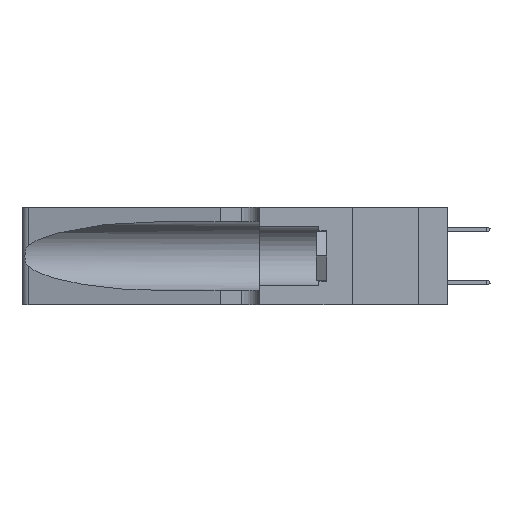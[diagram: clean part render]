
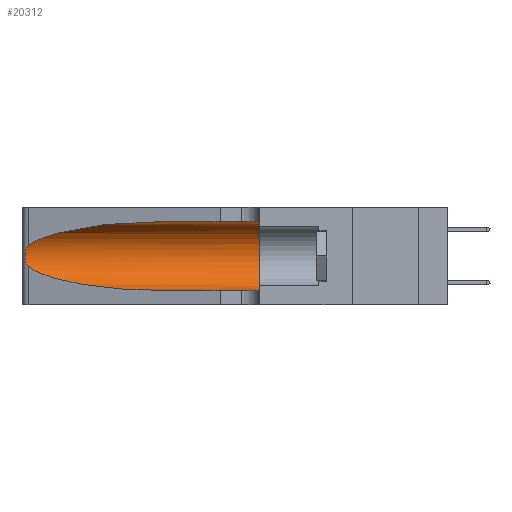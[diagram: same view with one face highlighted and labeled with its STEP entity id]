
A CAD part, left-side view. The second image highlights one B-rep face of the part: STEP entity #20312.
In plain terms, the highlighted cylindrical face has radius 3.308 mm (diameter 6.617 mm), a partial arc.
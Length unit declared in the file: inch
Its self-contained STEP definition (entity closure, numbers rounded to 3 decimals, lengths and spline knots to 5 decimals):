
#428 = VERTEX_POINT ( 'NONE', #33057 ) ;
#535 = ORIENTED_EDGE ( 'NONE', *, *, #45934, .F. ) ;
#1060 = CARTESIAN_POINT ( 'NONE',  ( 0.25639, 1.23186, 0.15144 ) ) ;
#3641 = CARTESIAN_POINT ( 'NONE',  ( 0.1305, 0.72297, 0.31525 ) ) ;
#3843 = LINE ( 'NONE', #36779, #40829 ) ;
#3960 = CARTESIAN_POINT ( 'NONE',  ( 0.1305, 0.35, 0.05475 ) ) ;
#4656 = CARTESIAN_POINT ( 'NONE',  ( 0.25639, 1.23184, 0.21858 ) ) ;
#4791 = VECTOR ( 'NONE', #8907, 39.37008 ) ;
#5279 = CARTESIAN_POINT ( 'NONE',  ( 0.25555, 1.22994, 0.2215 ) ) ;
#5611 = CARTESIAN_POINT ( 'NONE',  ( 0.18966, 0.96281, 0.31525 ) ) ;
#6118 = ORIENTED_EDGE ( 'NONE', *, *, #34752, .T. ) ;
#6640 = CARTESIAN_POINT ( 'NONE',  ( 0.1305, 0.35, 0.185 ) ) ;
#7784 = DIRECTION ( 'NONE',  ( 0., -1., 0. ) ) ;
#7878 = CARTESIAN_POINT ( 'NONE',  ( 0.25487, 1.22718, 0.14631 ) ) ;
#7932 = DIRECTION ( 'NONE',  ( 0., 0., -1. ) ) ;
#8340 = CARTESIAN_POINT ( 'NONE',  ( 0.1305, 0.72297, 0.05475 ) ) ;
#8907 = DIRECTION ( 'NONE',  ( 0., -1., 0. ) ) ;
#9810 = ORIENTED_EDGE ( 'NONE', *, *, #25348, .T. ) ;
#10190 = EDGE_LOOP ( 'NONE', ( #35758, #9810, #6118, #24271, #42509, #535 ) ) ;
#10231 = FACE_OUTER_BOUND ( 'NONE', #10190, .T. ) ;
#10929 = CARTESIAN_POINT ( 'NONE',  ( 0.1305, 0.72297, 0.05475 ) ) ;
#12458 = CARTESIAN_POINT ( 'NONE',  ( 0.25787, 1.23484, 0.2124 ) ) ;
#13278 = VERTEX_POINT ( 'NONE', #3641 ) ;
#15458 = CARTESIAN_POINT ( 'NONE',  ( 0.26075, 1.23896, 0.19203 ) ) ;
#15604 = CARTESIAN_POINT ( 'NONE',  ( 0.26075, 1.23896, 0.178 ) ) ;
#16070 = CARTESIAN_POINT ( 'NONE',  ( 0.25856, 1.23593, 0.16098 ) ) ;
#17024 = AXIS2_PLACEMENT_3D ( 'NONE', #6640, #39417, #32506 ) ;
#18526 = CARTESIAN_POINT ( 'NONE',  ( 0.2373, 1.15595, 0.08982 ) ) ;
#19727 = VERTEX_POINT ( 'NONE', #3960 ) ;
#20312 = ADVANCED_FACE ( 'NONE', ( #10231 ), #21423, .F. ) ;
#20934 = EDGE_CURVE ( 'NONE', #27615, #19727, #43351, .T. ) ;
#21423 = CYLINDRICAL_SURFACE ( 'NONE', #39854, 0.13025 ) ;
#22131 = CARTESIAN_POINT ( 'NONE',  ( 0.1305, 0.35, 0.31525 ) ) ;
#22502 = CARTESIAN_POINT ( 'NONE',  ( 0.25487, 1.22718, 0.14631 ) ) ;
#23610 = EDGE_CURVE ( 'NONE', #29507, #19727, #3843, .T. ) ;
#24271 = ORIENTED_EDGE ( 'NONE', *, *, #23610, .T. ) ;
#25348 = EDGE_CURVE ( 'NONE', #428, #28505, #37617, .T. ) ;
#26445 = CARTESIAN_POINT ( 'NONE',  ( 0.25487, 1.22718, 0.22369 ) ) ;
#26723 =( BOUNDED_CURVE ( )  B_SPLINE_CURVE ( 3, ( #7878, #18526, #44082, #8340 ),
 .UNSPECIFIED., .F., .F. ) 
 B_SPLINE_CURVE_WITH_KNOTS ( ( 4, 4 ),
 ( 3.44316, 4.71239 ),
 .UNSPECIFIED. ) 
 CURVE ( )  GEOMETRIC_REPRESENTATION_ITEM ( )  RATIONAL_B_SPLINE_CURVE ( ( 1., 0.87, 0.87, 1. ) ) 
 REPRESENTATION_ITEM ( '' )  );
#26768 = CARTESIAN_POINT ( 'NONE',  ( 0.26018, 1.23835, 0.19895 ) ) ;
#27615 = VERTEX_POINT ( 'NONE', #22131 ) ;
#28505 = VERTEX_POINT ( 'NONE', #44675 ) ;
#29507 = VERTEX_POINT ( 'NONE', #10929 ) ;
#30391 = CARTESIAN_POINT ( 'NONE',  ( 0.1305, 1.61858, 0.31525 ) ) ;
#32270 = LINE ( 'NONE', #30391, #4791 ) ;
#32506 = DIRECTION ( 'NONE',  ( 0., 0., 1. ) ) ;
#33057 = CARTESIAN_POINT ( 'NONE',  ( 0.25487, 1.22718, 0.22369 ) ) ;
#33923 = CARTESIAN_POINT ( 'NONE',  ( 0.26017, 1.23833, 0.17102 ) ) ;
#34752 = EDGE_CURVE ( 'NONE', #28505, #29507, #26723, .T. ) ;
#35692 = CARTESIAN_POINT ( 'NONE',  ( 0.1305, 1.61858, 0.185 ) ) ;
#35758 = ORIENTED_EDGE ( 'NONE', *, *, #40510, .T. ) ;
#36779 = CARTESIAN_POINT ( 'NONE',  ( 0.1305, 1.61858, 0.05475 ) ) ;
#36920 = CARTESIAN_POINT ( 'NONE',  ( 0.25854, 1.2359, 0.20912 ) ) ;
#37617 = B_SPLINE_CURVE_WITH_KNOTS ( 'NONE', 3,
 ( #26445, #5279, #4656, #12458, #36920, #26768, #15458, #15604, #33923, #16070, #43980, #1060, #40695, #22502 ),
 .UNSPECIFIED., .F., .F.,
 ( 4, 2, 2, 2, 2, 2, 4 ),
 ( 0., 0.00027, 0.00053, 0.00107, 0.0016, 0.00187, 0.00214 ),
 .UNSPECIFIED. ) ;
#38196 = CARTESIAN_POINT ( 'NONE',  ( 0.1305, 0.72297, 0.31525 ) ) ;
#39324 = DIRECTION ( 'NONE',  ( 0., -1., 0. ) ) ;
#39417 = DIRECTION ( 'NONE',  ( 0., 1., 0. ) ) ;
#39854 = AXIS2_PLACEMENT_3D ( 'NONE', #35692, #39324, #7932 ) ;
#40510 = EDGE_CURVE ( 'NONE', #13278, #428, #42521, .T. ) ;
#40695 = CARTESIAN_POINT ( 'NONE',  ( 0.25555, 1.22993, 0.14849 ) ) ;
#40829 = VECTOR ( 'NONE', #7784, 39.37008 ) ;
#42509 = ORIENTED_EDGE ( 'NONE', *, *, #20934, .F. ) ;
#42521 =( BOUNDED_CURVE ( )  B_SPLINE_CURVE ( 3, ( #38196, #5611, #45252, #44948 ),
 .UNSPECIFIED., .F., .T. ) 
 B_SPLINE_CURVE_WITH_KNOTS ( ( 4, 4 ),
 ( 1.5708, 2.84003 ),
 .UNSPECIFIED. ) 
 CURVE ( )  GEOMETRIC_REPRESENTATION_ITEM ( )  RATIONAL_B_SPLINE_CURVE ( ( 1., 0.87, 0.87, 1. ) ) 
 REPRESENTATION_ITEM ( '' )  );
#43351 = CIRCLE ( 'NONE', #17024, 0.13025 ) ;
#43980 = CARTESIAN_POINT ( 'NONE',  ( 0.25789, 1.23486, 0.15765 ) ) ;
#44082 = CARTESIAN_POINT ( 'NONE',  ( 0.18966, 0.96281, 0.05475 ) ) ;
#44675 = CARTESIAN_POINT ( 'NONE',  ( 0.25487, 1.22718, 0.14631 ) ) ;
#44948 = CARTESIAN_POINT ( 'NONE',  ( 0.25487, 1.22718, 0.22369 ) ) ;
#45252 = CARTESIAN_POINT ( 'NONE',  ( 0.2373, 1.15595, 0.28018 ) ) ;
#45934 = EDGE_CURVE ( 'NONE', #13278, #27615, #32270, .T. ) ;
